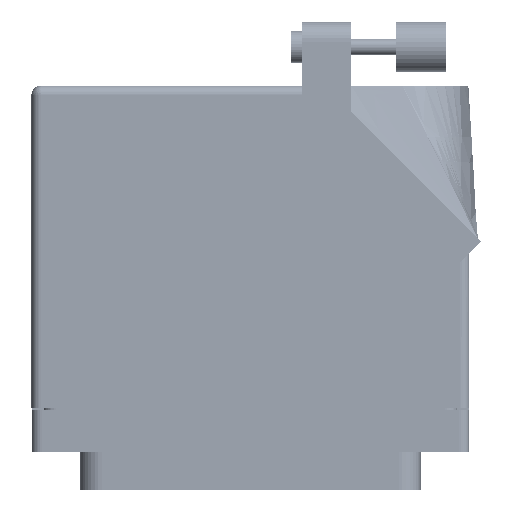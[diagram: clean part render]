
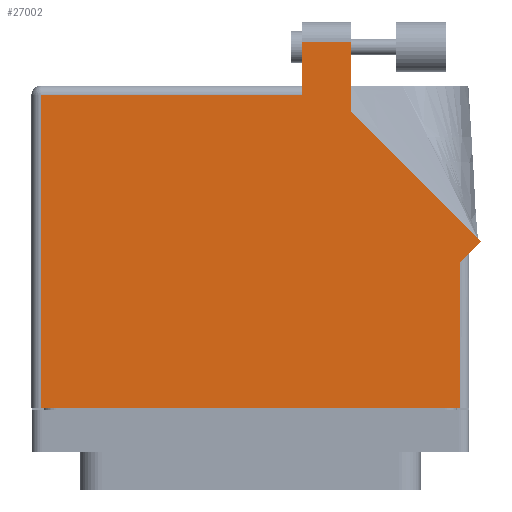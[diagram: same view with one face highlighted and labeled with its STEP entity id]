
A CAD part, front view. The second image highlights one B-rep face of the part: STEP entity #27002.
In plain terms, the highlighted face is planar.
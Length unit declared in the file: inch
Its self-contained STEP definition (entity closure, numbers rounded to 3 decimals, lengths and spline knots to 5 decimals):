
#761 = ORIENTED_EDGE ( 'NONE', *, *, #23708, .T. ) ;
#961 = VERTEX_POINT ( 'NONE', #47670 ) ;
#2741 = DIRECTION ( 'NONE',  ( 0., 1., 0. ) ) ;
#3092 = DIRECTION ( 'NONE',  ( -1., 0., 0. ) ) ;
#3131 = CARTESIAN_POINT ( 'NONE',  ( 1.3775, 0.88, 0.765 ) ) ;
#3357 = CARTESIAN_POINT ( 'NONE',  ( 0.6345, 1.76442, 0.765 ) ) ;
#3720 = LINE ( 'NONE', #59126, #77762 ) ;
#6170 = CARTESIAN_POINT ( 'NONE',  ( -1.3775, 1.868, 0.765 ) ) ;
#8080 = AXIS2_PLACEMENT_3D ( 'NONE', #38380, #9761, #80628 ) ;
#9761 = DIRECTION ( 'NONE',  ( 0., 0., -1. ) ) ;
#12519 = EDGE_LOOP ( 'NONE', ( #761, #39410, #48348, #20015, #67892, #38099, #78819, #71811, #44903 ) ) ;
#12802 = FACE_OUTER_BOUND ( 'NONE', #12519, .T. ) ;
#15411 = VECTOR ( 'NONE', #2741, 39.37008 ) ;
#16226 = DIRECTION ( 'NONE',  ( 0., -1., 0. ) ) ;
#20015 = ORIENTED_EDGE ( 'NONE', *, *, #65383, .T. ) ;
#23708 = EDGE_CURVE ( 'NONE', #52622, #68371, #39045, .T. ) ;
#27002 = ADVANCED_FACE ( 'NONE', ( #12802 ), #74080, .F. ) ;
#28382 = VERTEX_POINT ( 'NONE', #80637 ) ;
#29998 = VECTOR ( 'NONE', #53967, 39.37008 ) ;
#30693 = VECTOR ( 'NONE', #61131, 39.37008 ) ;
#31282 = VECTOR ( 'NONE', #56559, 39.37008 ) ;
#31659 = CARTESIAN_POINT ( 'NONE',  ( 0.6345, 1.76442, 0.765 ) ) ;
#31904 = CARTESIAN_POINT ( 'NONE',  ( -1.3155, -0.1, 0.765 ) ) ;
#31911 = LINE ( 'NONE', #3131, #53107 ) ;
#33548 = LINE ( 'NONE', #39207, #71687 ) ;
#36023 = CARTESIAN_POINT ( 'NONE',  ( -1.3775, -0.1, 0.765 ) ) ;
#38099 = ORIENTED_EDGE ( 'NONE', *, *, #74766, .T. ) ;
#38162 = CARTESIAN_POINT ( 'NONE',  ( 0.6345, 2.205, 0.765 ) ) ;
#38380 = CARTESIAN_POINT ( 'NONE',  ( -1.3775, 1.93, 0.765 ) ) ;
#38803 = EDGE_CURVE ( 'NONE', #68453, #79021, #50761, .T. ) ;
#39045 = LINE ( 'NONE', #3357, #15411 ) ;
#39112 = CARTESIAN_POINT ( 'NONE',  ( 1.3155, 0.818, 0.765 ) ) ;
#39207 = CARTESIAN_POINT ( 'NONE',  ( 0.3275, 2.205, 0.765 ) ) ;
#39410 = ORIENTED_EDGE ( 'NONE', *, *, #75298, .T. ) ;
#39594 = CARTESIAN_POINT ( 'NONE',  ( -1.3155, -0.1, 0.765 ) ) ;
#44903 = ORIENTED_EDGE ( 'NONE', *, *, #70837, .T. ) ;
#47670 = CARTESIAN_POINT ( 'NONE',  ( 1.44821, 0.95071, 0.765 ) ) ;
#48211 = LINE ( 'NONE', #36023, #75065 ) ;
#48348 = ORIENTED_EDGE ( 'NONE', *, *, #52532, .T. ) ;
#50761 = LINE ( 'NONE', #39594, #30693 ) ;
#52293 = CARTESIAN_POINT ( 'NONE',  ( 0.3275, 1.868, 0.765 ) ) ;
#52532 = EDGE_CURVE ( 'NONE', #78920, #73720, #3720, .T. ) ;
#52622 = VERTEX_POINT ( 'NONE', #31659 ) ;
#53107 = VECTOR ( 'NONE', #60456, 39.37008 ) ;
#53967 = DIRECTION ( 'NONE',  ( 0., 1., 0. ) ) ;
#56559 = DIRECTION ( 'NONE',  ( -1., 0., 0. ) ) ;
#57729 = LINE ( 'NONE', #64647, #86888 ) ;
#57767 = DIRECTION ( 'NONE',  ( -0.707, 0.707, 0. ) ) ;
#59126 = CARTESIAN_POINT ( 'NONE',  ( 0.3275, 1.93, 0.765 ) ) ;
#60456 = DIRECTION ( 'NONE',  ( 0.707, 0.707, 0. ) ) ;
#61131 = DIRECTION ( 'NONE',  ( 0., -1., 0. ) ) ;
#61697 = EDGE_CURVE ( 'NONE', #76782, #961, #31911, .T. ) ;
#64647 = CARTESIAN_POINT ( 'NONE',  ( 1.44821, 0.95071, 0.765 ) ) ;
#65383 = EDGE_CURVE ( 'NONE', #73720, #68453, #70542, .T. ) ;
#67547 = CARTESIAN_POINT ( 'NONE',  ( -1.3155, 1.868, 0.765 ) ) ;
#67892 = ORIENTED_EDGE ( 'NONE', *, *, #38803, .T. ) ;
#68371 = VERTEX_POINT ( 'NONE', #38162 ) ;
#68453 = VERTEX_POINT ( 'NONE', #67547 ) ;
#69016 = CARTESIAN_POINT ( 'NONE',  ( 1.3155, 0.88, 0.765 ) ) ;
#69099 = LINE ( 'NONE', #69016, #29998 ) ;
#70542 = LINE ( 'NONE', #6170, #31282 ) ;
#70837 = EDGE_CURVE ( 'NONE', #961, #52622, #57729, .T. ) ;
#70994 = DIRECTION ( 'NONE',  ( 1., 0., 0. ) ) ;
#71687 = VECTOR ( 'NONE', #3092, 39.37008 ) ;
#71811 = ORIENTED_EDGE ( 'NONE', *, *, #61697, .T. ) ;
#73720 = VERTEX_POINT ( 'NONE', #52293 ) ;
#74080 = PLANE ( 'NONE',  #8080 ) ;
#74766 = EDGE_CURVE ( 'NONE', #79021, #28382, #48211, .T. ) ;
#75065 = VECTOR ( 'NONE', #70994, 39.37008 ) ;
#75298 = EDGE_CURVE ( 'NONE', #68371, #78920, #33548, .T. ) ;
#76782 = VERTEX_POINT ( 'NONE', #39112 ) ;
#77762 = VECTOR ( 'NONE', #16226, 39.37008 ) ;
#78819 = ORIENTED_EDGE ( 'NONE', *, *, #91157, .T. ) ;
#78920 = VERTEX_POINT ( 'NONE', #85793 ) ;
#79021 = VERTEX_POINT ( 'NONE', #31904 ) ;
#80628 = DIRECTION ( 'NONE',  ( -1., 0., 0. ) ) ;
#80637 = CARTESIAN_POINT ( 'NONE',  ( 1.3155, -0.1, 0.765 ) ) ;
#85793 = CARTESIAN_POINT ( 'NONE',  ( 0.3275, 2.205, 0.765 ) ) ;
#86888 = VECTOR ( 'NONE', #57767, 39.37008 ) ;
#91157 = EDGE_CURVE ( 'NONE', #28382, #76782, #69099, .T. ) ;
